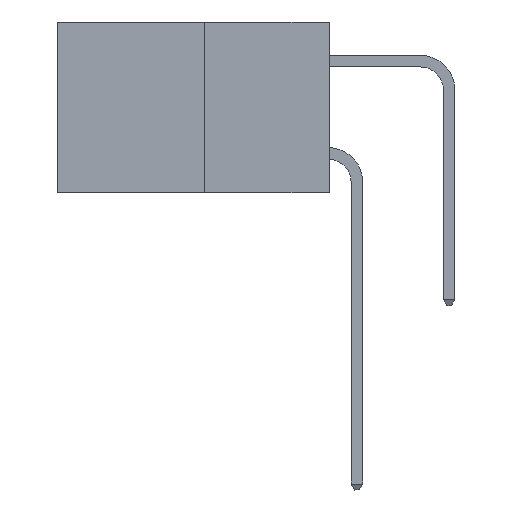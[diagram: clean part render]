
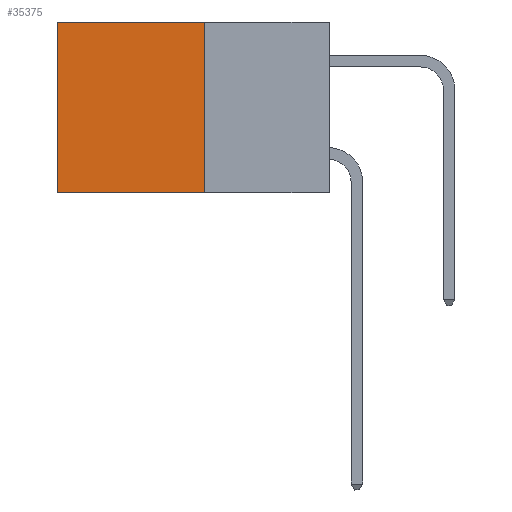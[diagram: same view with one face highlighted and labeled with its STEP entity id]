
A CAD part, left-side view. The second image highlights one B-rep face of the part: STEP entity #35375.
In plain terms, the highlighted planar face has unit normal (-1, 0, 0).
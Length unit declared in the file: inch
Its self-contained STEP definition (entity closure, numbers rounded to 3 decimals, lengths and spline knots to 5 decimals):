
#1239 = DIRECTION ( 'NONE',  ( 1., 0., 0. ) ) ;
#1701 = ORIENTED_EDGE ( 'NONE', *, *, #5243, .T. ) ;
#1950 = EDGE_CURVE ( 'NONE', #24856, #7241, #29791, .T. ) ;
#2072 = CARTESIAN_POINT ( 'NONE',  ( 0.277, 0.59, -0.37 ) ) ;
#2137 = ORIENTED_EDGE ( 'NONE', *, *, #1950, .F. ) ;
#3614 = DIRECTION ( 'NONE',  ( 0., 1., 0. ) ) ;
#5243 = EDGE_CURVE ( 'NONE', #24856, #17912, #17690, .T. ) ;
#5416 = CARTESIAN_POINT ( 'NONE',  ( 0.277, 0.27, -0.37 ) ) ;
#7238 = DIRECTION ( 'NONE',  ( 0., 0., -1. ) ) ;
#7241 = VERTEX_POINT ( 'NONE', #5416 ) ;
#9405 = FACE_OUTER_BOUND ( 'NONE', #25607, .T. ) ;
#9416 = PLANE ( 'NONE',  #14266 ) ;
#11607 = VERTEX_POINT ( 'NONE', #2072 ) ;
#14266 = AXIS2_PLACEMENT_3D ( 'NONE', #25783, #1239, #20466 ) ;
#15077 = VECTOR ( 'NONE', #3614, 39.37008 ) ;
#16542 = EDGE_CURVE ( 'NONE', #17912, #11607, #21561, .T. ) ;
#17690 = LINE ( 'NONE', #34596, #31311 ) ;
#17912 = VERTEX_POINT ( 'NONE', #27243 ) ;
#20466 = DIRECTION ( 'NONE',  ( 0., 0., -1. ) ) ;
#21561 = LINE ( 'NONE', #29284, #27079 ) ;
#24856 = VERTEX_POINT ( 'NONE', #28007 ) ;
#25607 = EDGE_LOOP ( 'NONE', ( #31622, #30336, #2137, #1701 ) ) ;
#25783 = CARTESIAN_POINT ( 'NONE',  ( 0.277, 0.27, -0.37 ) ) ;
#27079 = VECTOR ( 'NONE', #32039, 39.37008 ) ;
#27243 = CARTESIAN_POINT ( 'NONE',  ( 0.277, 0.59, 0. ) ) ;
#28007 = CARTESIAN_POINT ( 'NONE',  ( 0.277, 0.27, 0. ) ) ;
#28107 = CARTESIAN_POINT ( 'NONE',  ( 0.277, 0.27, -0.37 ) ) ;
#28924 = VECTOR ( 'NONE', #7238, 39.37008 ) ;
#29284 = CARTESIAN_POINT ( 'NONE',  ( 0.277, 0.59, -0.37 ) ) ;
#29791 = LINE ( 'NONE', #34373, #28924 ) ;
#30336 = ORIENTED_EDGE ( 'NONE', *, *, #34055, .F. ) ;
#30409 = LINE ( 'NONE', #28107, #15077 ) ;
#31311 = VECTOR ( 'NONE', #33715, 39.37008 ) ;
#31622 = ORIENTED_EDGE ( 'NONE', *, *, #16542, .T. ) ;
#32039 = DIRECTION ( 'NONE',  ( 0., 0., -1. ) ) ;
#33715 = DIRECTION ( 'NONE',  ( 0., 1., 0. ) ) ;
#34055 = EDGE_CURVE ( 'NONE', #7241, #11607, #30409, .T. ) ;
#34373 = CARTESIAN_POINT ( 'NONE',  ( 0.277, 0.27, -0.37 ) ) ;
#34596 = CARTESIAN_POINT ( 'NONE',  ( 0.277, 0.27, 0. ) ) ;
#35375 = ADVANCED_FACE ( 'NONE', ( #9405 ), #9416, .F. ) ;
